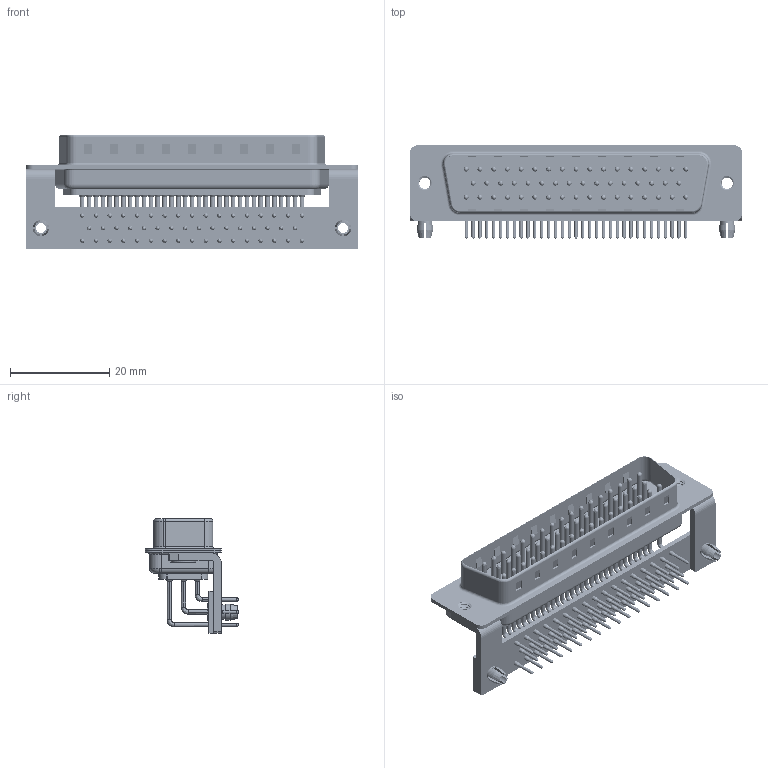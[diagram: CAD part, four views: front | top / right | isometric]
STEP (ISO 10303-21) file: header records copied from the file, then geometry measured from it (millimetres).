
FILE_DESCRIPTION (( 'STEP AP203' ), '1' );
FILE_NAME ('629-M50-240-GT3.STEP', '2018-09-25T23:43:59', ( '' ), ( '' ), 'SwSTEP 2.0', 'SolidWorks 2016', '' );
FILE_SCHEMA (( 'CONFIG_CONTROL_DESIGN' ));
Length unit declared in the file: millimetre
Products named in the file (11): 629M 4-40 Threaded Rivet_Stabilizer; 629M Stabilizer Bracket_50 Contacts; 629M Stabilizer Board_50 Contacts; 629M Housing_50 Contacts; 629M Board Lock_50 Contacts; 629M Shell Front_50 Contacts; 629-M50-240-GT3; 629M Shell Rear_50 Contacts; 629M Contact Row 1_50 Contacts; 629M Contact Row 2_50 Contacts; 629M Contact Row 3
Assembly tree (60 placements, depth 2):
  629-M50-240-GT3
    629M Housing_50 Contacts
    629M Shell Front_50 Contacts
    629M Shell Rear_50 Contacts
    629M Contact Row 1_50 Contacts  x17
    629M Contact Row 2_50 Contacts  x16
    629M Contact Row 3  x17
    629M 4-40 Threaded Rivet_Stabilizer  x2
    629M Stabilizer Bracket_50 Contacts  x2
    629M Stabilizer Board_50 Contacts
    629M Board Lock_50 Contacts  x2
Bounding box: 67 x 18.8 x 23.1 mm (x, y, z)
Volume: 5879.1 mm3; surface area: 15169.1 mm2
Topology: 60 solids, 60 shells, 6154 faces, 17267 edges, 11248 vertices
Faces by surface type: plane 3477, cylinder 2095, bspline 306, cone 220, torus 56
Entity records: 43614 total; most frequent: CARTESIAN_POINT 8499, DIRECTION 7205, ORIENTED_EDGE 6484, EDGE_CURVE 3242, AXIS2_PLACEMENT_3D 2711, VERTEX_POINT 2118, VECTOR 1783, LINE 1783
